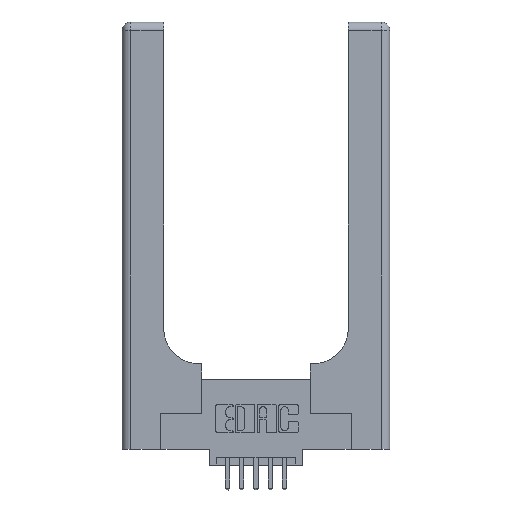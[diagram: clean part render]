
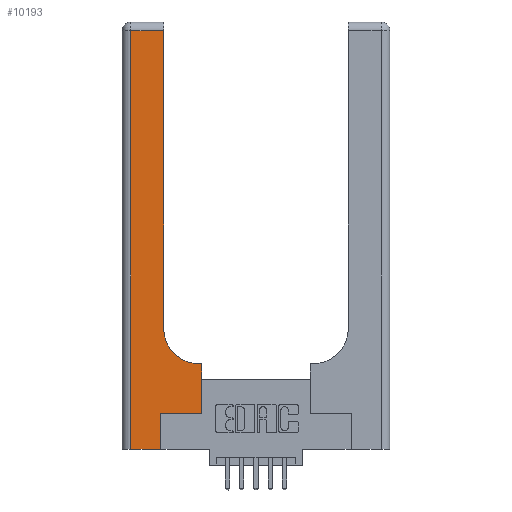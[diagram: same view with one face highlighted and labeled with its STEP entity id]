
A CAD part, top view. The second image highlights one B-rep face of the part: STEP entity #10193.
In plain terms, the highlighted planar face has unit normal (0, 0, 1).
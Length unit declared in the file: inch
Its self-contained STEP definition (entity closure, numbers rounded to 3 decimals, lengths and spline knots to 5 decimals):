
#120 = VECTOR ( 'NONE', #6852, 39.37008 ) ;
#342 = DIRECTION ( 'NONE',  ( 1., 0., 0. ) ) ;
#380 = VERTEX_POINT ( 'NONE', #3917 ) ;
#463 = VERTEX_POINT ( 'NONE', #8427 ) ;
#673 = CIRCLE ( 'NONE', #7443, 0.25 ) ;
#750 = DIRECTION ( 'NONE',  ( 0., 1., 0. ) ) ;
#896 = CARTESIAN_POINT ( 'NONE',  ( 0.06, 3., 0.37 ) ) ;
#966 = CARTESIAN_POINT ( 'NONE',  ( 0.2915, 3., 0.37 ) ) ;
#1292 = EDGE_LOOP ( 'NONE', ( #1969, #4792, #5694, #13550, #8928, #12678, #2522, #4819, #4118 ) ) ;
#1912 = VECTOR ( 'NONE', #13635, 39.37008 ) ;
#1969 = ORIENTED_EDGE ( 'NONE', *, *, #5213, .T. ) ;
#2383 = CARTESIAN_POINT ( 'NONE',  ( 0.2915, 0.85, 0.37 ) ) ;
#2522 = ORIENTED_EDGE ( 'NONE', *, *, #13591, .T. ) ;
#2577 = LINE ( 'NONE', #10104, #120 ) ;
#2588 = CARTESIAN_POINT ( 'NONE',  ( 0.2915, 2.94, 0.37 ) ) ;
#2591 = CARTESIAN_POINT ( 'NONE',  ( 0.5415, 0.85, 0.37 ) ) ;
#3038 = CARTESIAN_POINT ( 'NONE',  ( 0.269, 0., 0.37 ) ) ;
#3139 = EDGE_CURVE ( 'NONE', #9409, #463, #5404, .T. ) ;
#3387 = CARTESIAN_POINT ( 'NONE',  ( 0., 3., 0.37 ) ) ;
#3651 = VECTOR ( 'NONE', #750, 39.37008 ) ;
#3678 = CARTESIAN_POINT ( 'NONE',  ( 0., 0., 0.37 ) ) ;
#3835 = EDGE_CURVE ( 'NONE', #463, #8467, #4511, .T. ) ;
#3917 = CARTESIAN_POINT ( 'NONE',  ( 0.06, 2.94, 0.37 ) ) ;
#4118 = ORIENTED_EDGE ( 'NONE', *, *, #9194, .T. ) ;
#4319 = CARTESIAN_POINT ( 'NONE',  ( 0.5585, 0.25, 0.37 ) ) ;
#4511 = LINE ( 'NONE', #6217, #5378 ) ;
#4792 = ORIENTED_EDGE ( 'NONE', *, *, #11971, .T. ) ;
#4819 = ORIENTED_EDGE ( 'NONE', *, *, #9084, .T. ) ;
#4825 = VECTOR ( 'NONE', #6482, 39.37008 ) ;
#5062 = LINE ( 'NONE', #13043, #12489 ) ;
#5213 = EDGE_CURVE ( 'NONE', #8078, #12265, #14337, .T. ) ;
#5378 = VECTOR ( 'NONE', #10689, 39.37008 ) ;
#5404 = LINE ( 'NONE', #3038, #3651 ) ;
#5694 = ORIENTED_EDGE ( 'NONE', *, *, #11905, .T. ) ;
#5840 = AXIS2_PLACEMENT_3D ( 'NONE', #3387, #7708, #11049 ) ;
#6217 = CARTESIAN_POINT ( 'NONE',  ( 0.269, 0.25, 0.37 ) ) ;
#6462 = DIRECTION ( 'NONE',  ( 0., 1., 0. ) ) ;
#6482 = DIRECTION ( 'NONE',  ( 0., 1., 0. ) ) ;
#6487 = VERTEX_POINT ( 'NONE', #13356 ) ;
#6822 = VECTOR ( 'NONE', #8938, 39.37008 ) ;
#6852 = DIRECTION ( 'NONE',  ( -1., 0., 0. ) ) ;
#6910 = DIRECTION ( 'NONE',  ( 0., 0., -1. ) ) ;
#7375 = LINE ( 'NONE', #896, #11497 ) ;
#7443 = AXIS2_PLACEMENT_3D ( 'NONE', #2591, #6910, #342 ) ;
#7586 = CARTESIAN_POINT ( 'NONE',  ( 0.269, 0., 0.37 ) ) ;
#7708 = DIRECTION ( 'NONE',  ( 0., 0., -1. ) ) ;
#8058 = EDGE_CURVE ( 'NONE', #10792, #9409, #13829, .T. ) ;
#8078 = VERTEX_POINT ( 'NONE', #2383 ) ;
#8427 = CARTESIAN_POINT ( 'NONE',  ( 0.269, 0.25, 0.37 ) ) ;
#8467 = VERTEX_POINT ( 'NONE', #4319 ) ;
#8928 = ORIENTED_EDGE ( 'NONE', *, *, #3139, .T. ) ;
#8938 = DIRECTION ( 'NONE',  ( -1., 0., 0. ) ) ;
#9084 = EDGE_CURVE ( 'NONE', #11119, #6487, #2577, .T. ) ;
#9194 = EDGE_CURVE ( 'NONE', #6487, #8078, #673, .T. ) ;
#9251 = LINE ( 'NONE', #10980, #6822 ) ;
#9409 = VERTEX_POINT ( 'NONE', #7586 ) ;
#9821 = DIRECTION ( 'NONE',  ( 0., -1., 0. ) ) ;
#10104 = CARTESIAN_POINT ( 'NONE',  ( 0.2915, 0.6, 0.37 ) ) ;
#10193 = ADVANCED_FACE ( 'NONE', ( #12052 ), #13292, .F. ) ;
#10224 = CARTESIAN_POINT ( 'NONE',  ( 0.5585, 0.6, 0.37 ) ) ;
#10689 = DIRECTION ( 'NONE',  ( 1., 0., 0. ) ) ;
#10792 = VERTEX_POINT ( 'NONE', #14125 ) ;
#10980 = CARTESIAN_POINT ( 'NONE',  ( 0., 2.94, 0.37 ) ) ;
#11049 = DIRECTION ( 'NONE',  ( -1., 0., 0. ) ) ;
#11119 = VERTEX_POINT ( 'NONE', #10224 ) ;
#11497 = VECTOR ( 'NONE', #9821, 39.37008 ) ;
#11905 = EDGE_CURVE ( 'NONE', #380, #10792, #7375, .T. ) ;
#11971 = EDGE_CURVE ( 'NONE', #12265, #380, #9251, .T. ) ;
#12052 = FACE_OUTER_BOUND ( 'NONE', #1292, .T. ) ;
#12265 = VERTEX_POINT ( 'NONE', #2588 ) ;
#12489 = VECTOR ( 'NONE', #6462, 39.37008 ) ;
#12678 = ORIENTED_EDGE ( 'NONE', *, *, #3835, .T. ) ;
#13043 = CARTESIAN_POINT ( 'NONE',  ( 0.5585, 0.25, 0.37 ) ) ;
#13292 = PLANE ( 'NONE',  #5840 ) ;
#13356 = CARTESIAN_POINT ( 'NONE',  ( 0.5415, 0.6, 0.37 ) ) ;
#13550 = ORIENTED_EDGE ( 'NONE', *, *, #8058, .T. ) ;
#13591 = EDGE_CURVE ( 'NONE', #8467, #11119, #5062, .T. ) ;
#13635 = DIRECTION ( 'NONE',  ( 1., 0., 0. ) ) ;
#13829 = LINE ( 'NONE', #3678, #1912 ) ;
#14125 = CARTESIAN_POINT ( 'NONE',  ( 0.06, 0., 0.37 ) ) ;
#14337 = LINE ( 'NONE', #966, #4825 ) ;
